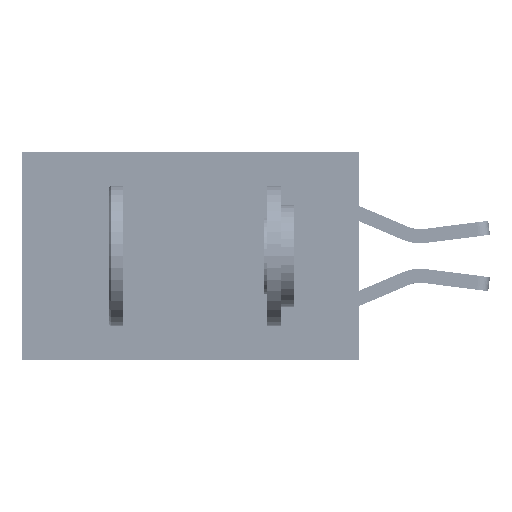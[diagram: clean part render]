
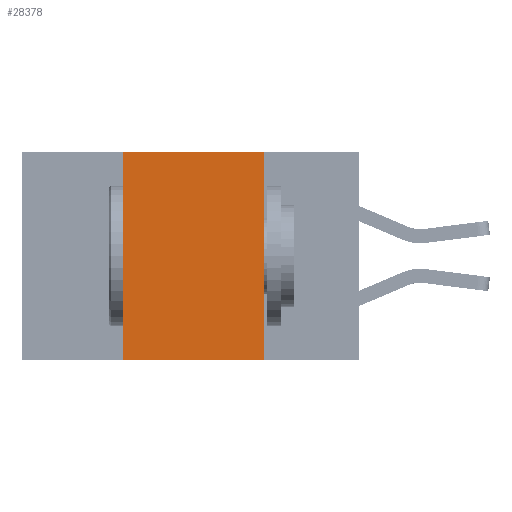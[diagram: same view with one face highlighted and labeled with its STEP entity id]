
A CAD part, left-side view. The second image highlights one B-rep face of the part: STEP entity #28378.
In plain terms, the highlighted planar face has unit normal (-1, 0, 0).
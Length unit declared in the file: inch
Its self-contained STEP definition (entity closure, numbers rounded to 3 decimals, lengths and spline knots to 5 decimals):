
#9335 = EDGE_CURVE ( 'NONE', #27569, #40776, #24904, .T. ) ;
#9742 = VECTOR ( 'NONE', #25422, 39.37008 ) ;
#10321 = VERTEX_POINT ( 'NONE', #21057 ) ;
#14606 = CARTESIAN_POINT ( 'NONE',  ( 0., 0.6, 0. ) ) ;
#15443 = ORIENTED_EDGE ( 'NONE', *, *, #35193, .T. ) ;
#16550 = DIRECTION ( 'NONE',  ( 0., 0., -1. ) ) ;
#16652 = CARTESIAN_POINT ( 'NONE',  ( 0., 0.42, -0.37 ) ) ;
#17225 = CARTESIAN_POINT ( 'NONE',  ( 0., 0.6, 0. ) ) ;
#17552 = CARTESIAN_POINT ( 'NONE',  ( 0., 0.42, 0. ) ) ;
#18130 = DIRECTION ( 'NONE',  ( 1., 0., 0. ) ) ;
#18374 = AXIS2_PLACEMENT_3D ( 'NONE', #14606, #18130, #42827 ) ;
#19159 = DIRECTION ( 'NONE',  ( 0., 0., 1. ) ) ;
#21057 = CARTESIAN_POINT ( 'NONE',  ( 0., 0.17, 0. ) ) ;
#21085 = EDGE_CURVE ( 'NONE', #40776, #10321, #42740, .T. ) ;
#21902 = CARTESIAN_POINT ( 'NONE',  ( 0., 0.6, -0.37 ) ) ;
#21990 = VECTOR ( 'NONE', #16550, 39.37008 ) ;
#22048 = EDGE_LOOP ( 'NONE', ( #41327, #44043, #32636, #15443 ) ) ;
#23085 = LINE ( 'NONE', #37552, #21990 ) ;
#23177 = VERTEX_POINT ( 'NONE', #43924 ) ;
#24904 = LINE ( 'NONE', #43852, #42599 ) ;
#25422 = DIRECTION ( 'NONE',  ( 0., -1., 0. ) ) ;
#27569 = VERTEX_POINT ( 'NONE', #16652 ) ;
#28378 = ADVANCED_FACE ( 'NONE', ( #29895 ), #35732, .F. ) ;
#29895 = FACE_OUTER_BOUND ( 'NONE', #22048, .T. ) ;
#32636 = ORIENTED_EDGE ( 'NONE', *, *, #9335, .F. ) ;
#33353 = VECTOR ( 'NONE', #45466, 39.37008 ) ;
#35193 = EDGE_CURVE ( 'NONE', #27569, #23177, #37939, .T. ) ;
#35732 = PLANE ( 'NONE',  #18374 ) ;
#37552 = CARTESIAN_POINT ( 'NONE',  ( 0., 0.17, 0. ) ) ;
#37939 = LINE ( 'NONE', #21902, #9742 ) ;
#39976 = EDGE_CURVE ( 'NONE', #10321, #23177, #23085, .T. ) ;
#40776 = VERTEX_POINT ( 'NONE', #17552 ) ;
#41327 = ORIENTED_EDGE ( 'NONE', *, *, #39976, .F. ) ;
#42599 = VECTOR ( 'NONE', #19159, 39.37008 ) ;
#42740 = LINE ( 'NONE', #17225, #33353 ) ;
#42827 = DIRECTION ( 'NONE',  ( 0., 0., -1. ) ) ;
#43852 = CARTESIAN_POINT ( 'NONE',  ( 0., 0.42, 0. ) ) ;
#43924 = CARTESIAN_POINT ( 'NONE',  ( 0., 0.17, -0.37 ) ) ;
#44043 = ORIENTED_EDGE ( 'NONE', *, *, #21085, .F. ) ;
#45466 = DIRECTION ( 'NONE',  ( 0., -1., 0. ) ) ;
